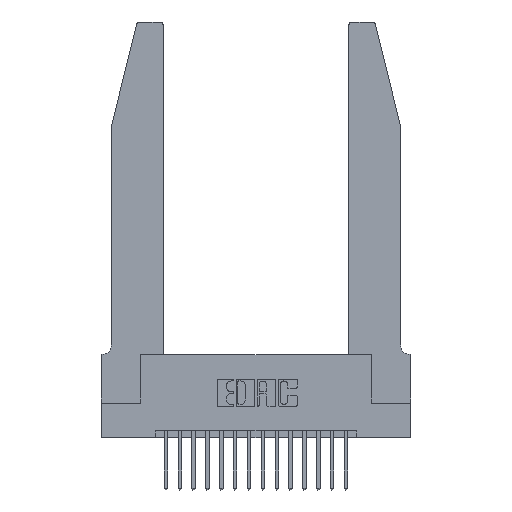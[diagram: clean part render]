
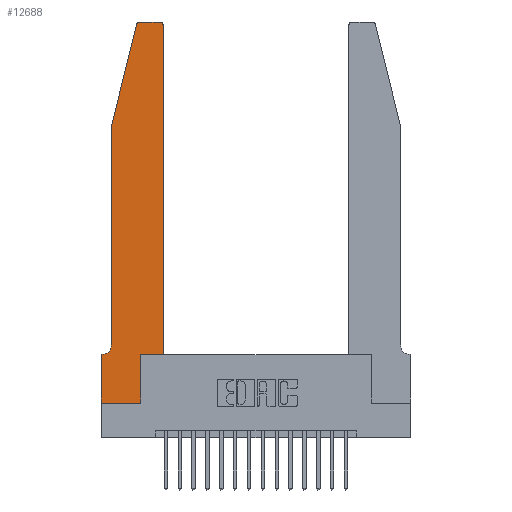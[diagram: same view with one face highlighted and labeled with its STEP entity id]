
A CAD part, top view. The second image highlights one B-rep face of the part: STEP entity #12688.
In plain terms, the highlighted planar face has unit normal (0, 0, 1).
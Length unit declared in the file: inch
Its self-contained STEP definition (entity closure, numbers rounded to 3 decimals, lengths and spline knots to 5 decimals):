
#270 = LINE ( 'NONE', #1055, #3509 ) ;
#500 = DIRECTION ( 'NONE',  ( 1., 0., 0. ) ) ;
#512 = CARTESIAN_POINT ( 'NONE',  ( 0.4505, 0.35, 0.37 ) ) ;
#628 = EDGE_CURVE ( 'NONE', #8084, #7670, #270, .T. ) ;
#657 = CARTESIAN_POINT ( 'NONE',  ( 0.4505, 2.72, 0.37 ) ) ;
#806 = DIRECTION ( 'NONE',  ( -1., 0., 0. ) ) ;
#964 = VECTOR ( 'NONE', #806, 39.37008 ) ;
#978 = VERTEX_POINT ( 'NONE', #16694 ) ;
#993 = ORIENTED_EDGE ( 'NONE', *, *, #6615, .T. ) ;
#1055 = CARTESIAN_POINT ( 'NONE',  ( 0., 0., 0.37 ) ) ;
#1522 = EDGE_CURVE ( 'NONE', #7670, #12247, #9332, .T. ) ;
#1621 = CARTESIAN_POINT ( 'NONE',  ( 0.2865, 0.35, 0.37 ) ) ;
#1773 = CIRCLE ( 'NONE', #14160, 0.03 ) ;
#1870 = ORIENTED_EDGE ( 'NONE', *, *, #15426, .T. ) ;
#1973 = DIRECTION ( 'NONE',  ( 0., -1., 0. ) ) ;
#2094 = VERTEX_POINT ( 'NONE', #1621 ) ;
#2231 = CARTESIAN_POINT ( 'NONE',  ( 0.25487, 2.72718, 0.37 ) ) ;
#2577 = ORIENTED_EDGE ( 'NONE', *, *, #7552, .T. ) ;
#2646 = CARTESIAN_POINT ( 'NONE',  ( 0.284, 2.75, 0.37 ) ) ;
#3343 = ORIENTED_EDGE ( 'NONE', *, *, #9811, .T. ) ;
#3480 = CARTESIAN_POINT ( 'NONE',  ( 0.0755, 2., 0.37 ) ) ;
#3509 = VECTOR ( 'NONE', #13176, 39.37008 ) ;
#3677 = EDGE_CURVE ( 'NONE', #2094, #5676, #8965, .T. ) ;
#3846 = VERTEX_POINT ( 'NONE', #657 ) ;
#4117 = CARTESIAN_POINT ( 'NONE',  ( 0.2865, 0.35, 0.37 ) ) ;
#4524 = CIRCLE ( 'NONE', #16280, 0.03 ) ;
#4554 = VECTOR ( 'NONE', #7576, 39.37008 ) ;
#4647 = PLANE ( 'NONE',  #9920 ) ;
#5357 = LINE ( 'NONE', #19388, #12742 ) ;
#5511 = EDGE_CURVE ( 'NONE', #3846, #6318, #1773, .T. ) ;
#5660 = DIRECTION ( 'NONE',  ( 0., 1., 0. ) ) ;
#5676 = VERTEX_POINT ( 'NONE', #16541 ) ;
#5822 = CARTESIAN_POINT ( 'NONE',  ( 0., 0., 0.37 ) ) ;
#5894 = DIRECTION ( 'NONE',  ( 0., 0., 1. ) ) ;
#5983 = CARTESIAN_POINT ( 'NONE',  ( 0.0055, 0.35, 0.37 ) ) ;
#6002 = ORIENTED_EDGE ( 'NONE', *, *, #3677, .T. ) ;
#6318 = VERTEX_POINT ( 'NONE', #15324 ) ;
#6615 = EDGE_CURVE ( 'NONE', #12247, #2094, #8400, .T. ) ;
#6811 = EDGE_CURVE ( 'NONE', #6318, #6932, #9080, .T. ) ;
#6932 = VERTEX_POINT ( 'NONE', #2646 ) ;
#7297 = VERTEX_POINT ( 'NONE', #2231 ) ;
#7380 = ORIENTED_EDGE ( 'NONE', *, *, #5511, .T. ) ;
#7440 = CARTESIAN_POINT ( 'NONE',  ( 0.4505, 0.35, 0.37 ) ) ;
#7552 = EDGE_CURVE ( 'NONE', #7297, #10273, #5357, .T. ) ;
#7576 = DIRECTION ( 'NONE',  ( 1., 0., 0. ) ) ;
#7670 = VERTEX_POINT ( 'NONE', #15239 ) ;
#7848 = EDGE_CURVE ( 'NONE', #18975, #8084, #16504, .T. ) ;
#7956 = VECTOR ( 'NONE', #5660, 39.37008 ) ;
#8084 = VERTEX_POINT ( 'NONE', #10381 ) ;
#8400 = LINE ( 'NONE', #4117, #7956 ) ;
#8448 = CARTESIAN_POINT ( 'NONE',  ( 0.2605, 2.75, 0.37 ) ) ;
#8460 = DIRECTION ( 'NONE',  ( 1., 0., 0. ) ) ;
#8853 = CARTESIAN_POINT ( 'NONE',  ( 0.0055, 0.42, 0.37 ) ) ;
#8965 = LINE ( 'NONE', #7440, #4554 ) ;
#8993 = DIRECTION ( 'NONE',  ( -0.239, -0.971, 0. ) ) ;
#9080 = LINE ( 'NONE', #8448, #964 ) ;
#9113 = CARTESIAN_POINT ( 'NONE',  ( 0., 0.35, 0.37 ) ) ;
#9239 = VECTOR ( 'NONE', #18608, 39.37008 ) ;
#9332 = LINE ( 'NONE', #5822, #10247 ) ;
#9625 = DIRECTION ( 'NONE',  ( 0., 0., 1. ) ) ;
#9735 = CARTESIAN_POINT ( 'NONE',  ( 0.0755, 0.35, 0.37 ) ) ;
#9773 = EDGE_CURVE ( 'NONE', #10273, #978, #12401, .T. ) ;
#9811 = EDGE_CURVE ( 'NONE', #6932, #7297, #4524, .T. ) ;
#9920 = AXIS2_PLACEMENT_3D ( 'NONE', #9113, #19511, #10595 ) ;
#10247 = VECTOR ( 'NONE', #8460, 39.37008 ) ;
#10273 = VERTEX_POINT ( 'NONE', #3480 ) ;
#10324 = DIRECTION ( 'NONE',  ( -1., 0., 0. ) ) ;
#10381 = CARTESIAN_POINT ( 'NONE',  ( 0., 0.35, 0.37 ) ) ;
#10595 = DIRECTION ( 'NONE',  ( 1., 0., 0. ) ) ;
#10617 = ORIENTED_EDGE ( 'NONE', *, *, #628, .T. ) ;
#12153 = CIRCLE ( 'NONE', #16363, 0.07 ) ;
#12247 = VERTEX_POINT ( 'NONE', #16894 ) ;
#12401 = LINE ( 'NONE', #14005, #16398 ) ;
#12688 = ADVANCED_FACE ( 'NONE', ( #12777 ), #4647, .T. ) ;
#12742 = VECTOR ( 'NONE', #8993, 39.37008 ) ;
#12777 = FACE_OUTER_BOUND ( 'NONE', #18853, .T. ) ;
#13176 = DIRECTION ( 'NONE',  ( 0., -1., 0. ) ) ;
#13651 = LINE ( 'NONE', #512, #9239 ) ;
#14005 = CARTESIAN_POINT ( 'NONE',  ( 0.0755, 2., 0.37 ) ) ;
#14160 = AXIS2_PLACEMENT_3D ( 'NONE', #14760, #5894, #16279 ) ;
#14760 = CARTESIAN_POINT ( 'NONE',  ( 0.4205, 2.72, 0.37 ) ) ;
#15056 = ORIENTED_EDGE ( 'NONE', *, *, #6811, .T. ) ;
#15239 = CARTESIAN_POINT ( 'NONE',  ( 0., 0., 0.37 ) ) ;
#15324 = CARTESIAN_POINT ( 'NONE',  ( 0.4205, 2.75, 0.37 ) ) ;
#15407 = ORIENTED_EDGE ( 'NONE', *, *, #7848, .T. ) ;
#15426 = EDGE_CURVE ( 'NONE', #5676, #3846, #13651, .T. ) ;
#16032 = VECTOR ( 'NONE', #17252, 39.37008 ) ;
#16279 = DIRECTION ( 'NONE',  ( 1., 0., 0. ) ) ;
#16280 = AXIS2_PLACEMENT_3D ( 'NONE', #18529, #9625, #500 ) ;
#16363 = AXIS2_PLACEMENT_3D ( 'NONE', #8853, #19235, #10324 ) ;
#16398 = VECTOR ( 'NONE', #1973, 39.37008 ) ;
#16504 = LINE ( 'NONE', #9735, #16032 ) ;
#16541 = CARTESIAN_POINT ( 'NONE',  ( 0.4505, 0.35, 0.37 ) ) ;
#16694 = CARTESIAN_POINT ( 'NONE',  ( 0.0755, 0.42, 0.37 ) ) ;
#16894 = CARTESIAN_POINT ( 'NONE',  ( 0.2865, 0., 0.37 ) ) ;
#17252 = DIRECTION ( 'NONE',  ( -1., 0., 0. ) ) ;
#17809 = EDGE_CURVE ( 'NONE', #978, #18975, #12153, .T. ) ;
#18052 = ORIENTED_EDGE ( 'NONE', *, *, #9773, .T. ) ;
#18298 = ORIENTED_EDGE ( 'NONE', *, *, #1522, .T. ) ;
#18514 = ORIENTED_EDGE ( 'NONE', *, *, #17809, .T. ) ;
#18529 = CARTESIAN_POINT ( 'NONE',  ( 0.284, 2.72, 0.37 ) ) ;
#18608 = DIRECTION ( 'NONE',  ( 0., 1., 0. ) ) ;
#18853 = EDGE_LOOP ( 'NONE', ( #15056, #3343, #2577, #18052, #18514, #15407, #10617, #18298, #993, #6002, #1870, #7380 ) ) ;
#18975 = VERTEX_POINT ( 'NONE', #5983 ) ;
#19235 = DIRECTION ( 'NONE',  ( 0., 0., -1. ) ) ;
#19388 = CARTESIAN_POINT ( 'NONE',  ( 0.0755, 2., 0.37 ) ) ;
#19511 = DIRECTION ( 'NONE',  ( 0., 0., 1. ) ) ;
